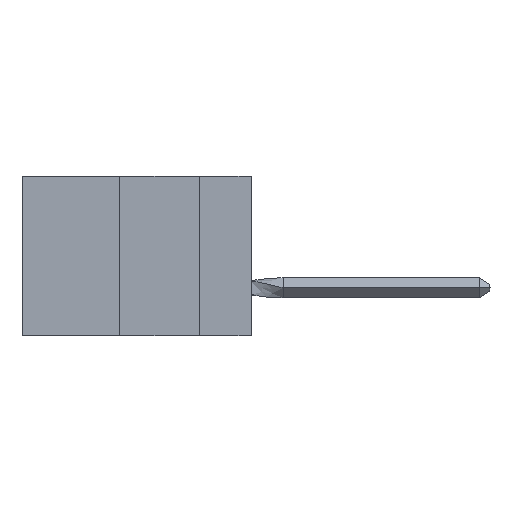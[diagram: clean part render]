
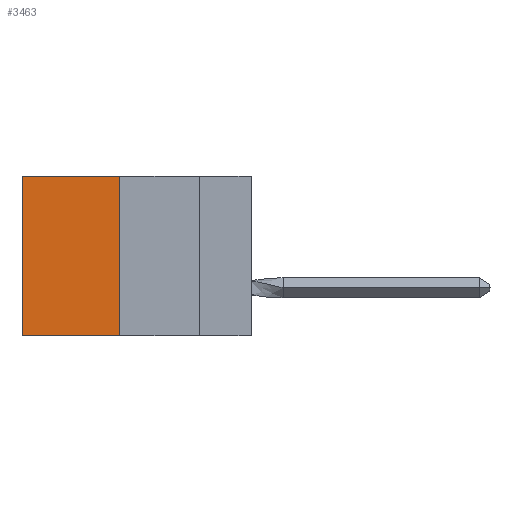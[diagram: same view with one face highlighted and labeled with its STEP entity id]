
A CAD part, left-side view. The second image highlights one B-rep face of the part: STEP entity #3463.
In plain terms, the highlighted planar face has unit normal (-1, 0, 0).
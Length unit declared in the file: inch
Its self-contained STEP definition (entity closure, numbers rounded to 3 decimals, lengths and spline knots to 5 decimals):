
#179 = LINE ( 'NONE', #1609, #9177 ) ;
#563 = ORIENTED_EDGE ( 'NONE', *, *, #6177, .F. ) ;
#1042 = LINE ( 'NONE', #11651, #19549 ) ;
#1570 = CARTESIAN_POINT ( 'NONE',  ( 0.305, 0.413, 0. ) ) ;
#1609 = CARTESIAN_POINT ( 'NONE',  ( 0.305, 0.413, -0.5 ) ) ;
#1778 = VECTOR ( 'NONE', #4445, 39.37008 ) ;
#1822 = ORIENTED_EDGE ( 'NONE', *, *, #14685, .T. ) ;
#1919 = AXIS2_PLACEMENT_3D ( 'NONE', #14049, #12329, #10956 ) ;
#2452 = EDGE_LOOP ( 'NONE', ( #1822, #12680, #563, #2579 ) ) ;
#2579 = ORIENTED_EDGE ( 'NONE', *, *, #14577, .T. ) ;
#3140 = LINE ( 'NONE', #8939, #15081 ) ;
#3463 = ADVANCED_FACE ( 'NONE', ( #13651 ), #4457, .F. ) ;
#4340 = CARTESIAN_POINT ( 'NONE',  ( 0.305, 0.72, -0.5 ) ) ;
#4445 = DIRECTION ( 'NONE',  ( 0., 1., 0. ) ) ;
#4457 = PLANE ( 'NONE',  #1919 ) ;
#4601 = VERTEX_POINT ( 'NONE', #5748 ) ;
#5748 = CARTESIAN_POINT ( 'NONE',  ( 0.305, 0.72, 0. ) ) ;
#6177 = EDGE_CURVE ( 'NONE', #8189, #7500, #1042, .T. ) ;
#6888 = LINE ( 'NONE', #18158, #1778 ) ;
#7500 = VERTEX_POINT ( 'NONE', #9773 ) ;
#8189 = VERTEX_POINT ( 'NONE', #1570 ) ;
#8939 = CARTESIAN_POINT ( 'NONE',  ( 0.305, 0.72, -0.5 ) ) ;
#9177 = VECTOR ( 'NONE', #11027, 39.37008 ) ;
#9773 = CARTESIAN_POINT ( 'NONE',  ( 0.305, 0.413, -0.5 ) ) ;
#10956 = DIRECTION ( 'NONE',  ( 0., 0., -1. ) ) ;
#11027 = DIRECTION ( 'NONE',  ( 0., 1., 0. ) ) ;
#11651 = CARTESIAN_POINT ( 'NONE',  ( 0.305, 0.413, -0.5 ) ) ;
#12329 = DIRECTION ( 'NONE',  ( 1., 0., 0. ) ) ;
#12590 = EDGE_CURVE ( 'NONE', #7500, #18422, #179, .T. ) ;
#12680 = ORIENTED_EDGE ( 'NONE', *, *, #12590, .F. ) ;
#13651 = FACE_OUTER_BOUND ( 'NONE', #2452, .T. ) ;
#14049 = CARTESIAN_POINT ( 'NONE',  ( 0.305, 0.413, -0.5 ) ) ;
#14524 = DIRECTION ( 'NONE',  ( 0., 0., -1. ) ) ;
#14577 = EDGE_CURVE ( 'NONE', #8189, #4601, #6888, .T. ) ;
#14685 = EDGE_CURVE ( 'NONE', #4601, #18422, #3140, .T. ) ;
#15081 = VECTOR ( 'NONE', #19825, 39.37008 ) ;
#18158 = CARTESIAN_POINT ( 'NONE',  ( 0.305, 0.413, 0. ) ) ;
#18422 = VERTEX_POINT ( 'NONE', #4340 ) ;
#19549 = VECTOR ( 'NONE', #14524, 39.37008 ) ;
#19825 = DIRECTION ( 'NONE',  ( 0., 0., -1. ) ) ;
